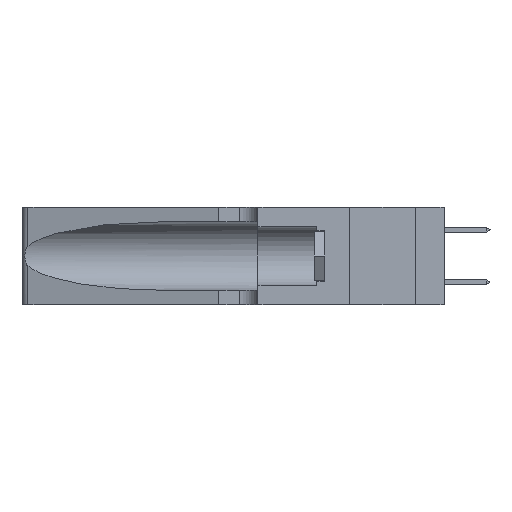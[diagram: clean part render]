
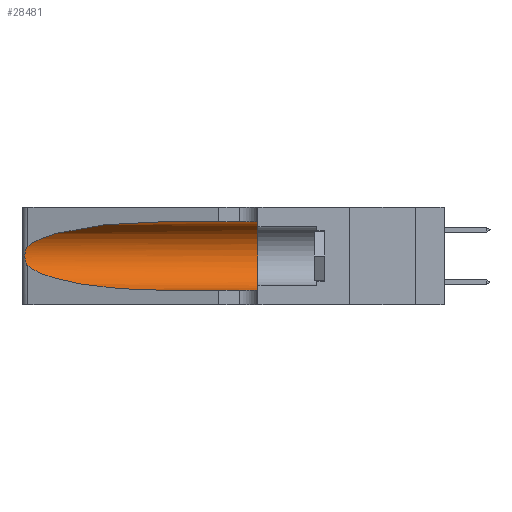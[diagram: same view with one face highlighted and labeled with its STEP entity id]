
A CAD part, left-side view. The second image highlights one B-rep face of the part: STEP entity #28481.
In plain terms, the highlighted cylindrical face has radius 3.308 mm (diameter 6.617 mm), a partial arc.
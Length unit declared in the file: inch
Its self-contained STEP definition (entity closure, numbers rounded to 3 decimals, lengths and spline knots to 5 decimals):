
#834 = DIRECTION ( 'NONE',  ( 0., -1., 0. ) ) ;
#1229 = VERTEX_POINT ( 'NONE', #6475 ) ;
#1246 = CARTESIAN_POINT ( 'NONE',  ( 0.25789, 1.23486, 0.15765 ) ) ;
#1828 = AXIS2_PLACEMENT_3D ( 'NONE', #7592, #24608, #10035 ) ;
#1978 = CARTESIAN_POINT ( 'NONE',  ( 0.1305, 0.35, 0.05475 ) ) ;
#2209 = DIRECTION ( 'NONE',  ( 0., 0., -1. ) ) ;
#2484 = AXIS2_PLACEMENT_3D ( 'NONE', #21669, #7104, #2209 ) ;
#3132 = CARTESIAN_POINT ( 'NONE',  ( 0.18966, 0.96281, 0.05475 ) ) ;
#3680 = CARTESIAN_POINT ( 'NONE',  ( 0.25555, 1.22993, 0.14849 ) ) ;
#4368 = VERTEX_POINT ( 'NONE', #24824 ) ;
#4526 = VECTOR ( 'NONE', #834, 39.37008 ) ;
#6027 = CARTESIAN_POINT ( 'NONE',  ( 0.25555, 1.22994, 0.2215 ) ) ;
#6126 = CARTESIAN_POINT ( 'NONE',  ( 0.25487, 1.22718, 0.22369 ) ) ;
#6475 = CARTESIAN_POINT ( 'NONE',  ( 0.25487, 1.22718, 0.22369 ) ) ;
#7104 = DIRECTION ( 'NONE',  ( 0., -1., 0. ) ) ;
#7253 = EDGE_CURVE ( 'NONE', #24562, #30715, #19856, .T. ) ;
#7592 = CARTESIAN_POINT ( 'NONE',  ( 0.1305, 0.35, 0.185 ) ) ;
#8226 = CARTESIAN_POINT ( 'NONE',  ( 0.25487, 1.22718, 0.14631 ) ) ;
#8473 = CARTESIAN_POINT ( 'NONE',  ( 0.25787, 1.23484, 0.2124 ) ) ;
#9405 = ORIENTED_EDGE ( 'NONE', *, *, #22318, .T. ) ;
#10035 = DIRECTION ( 'NONE',  ( 0., 0., 1. ) ) ;
#10339 = CARTESIAN_POINT ( 'NONE',  ( 0.1305, 0.72297, 0.31525 ) ) ;
#10905 = CARTESIAN_POINT ( 'NONE',  ( 0.26018, 1.23835, 0.19895 ) ) ;
#10991 = LINE ( 'NONE', #15040, #4526 ) ;
#11026 = CARTESIAN_POINT ( 'NONE',  ( 0.1305, 1.61858, 0.05475 ) ) ;
#12783 = CARTESIAN_POINT ( 'NONE',  ( 0.25487, 1.22718, 0.14631 ) ) ;
#12933 =( BOUNDED_CURVE ( )  B_SPLINE_CURVE ( 3, ( #12783, #24935, #3132, #20110 ),
 .UNSPECIFIED., .F., .F. ) 
 B_SPLINE_CURVE_WITH_KNOTS ( ( 4, 4 ),
 ( 3.44316, 4.71239 ),
 .UNSPECIFIED. ) 
 CURVE ( )  GEOMETRIC_REPRESENTATION_ITEM ( )  RATIONAL_B_SPLINE_CURVE ( ( 1., 0.87, 0.87, 1. ) ) 
 REPRESENTATION_ITEM ( '' )  );
#13247 = ORIENTED_EDGE ( 'NONE', *, *, #28868, .T. ) ;
#13335 = CARTESIAN_POINT ( 'NONE',  ( 0.26075, 1.23896, 0.178 ) ) ;
#13564 = EDGE_CURVE ( 'NONE', #16628, #24562, #10991, .T. ) ;
#15019 = LINE ( 'NONE', #11026, #21523 ) ;
#15040 = CARTESIAN_POINT ( 'NONE',  ( 0.1305, 1.61858, 0.31525 ) ) ;
#15261 = ORIENTED_EDGE ( 'NONE', *, *, #13564, .F. ) ;
#15773 = CARTESIAN_POINT ( 'NONE',  ( 0.18966, 0.96281, 0.31525 ) ) ;
#15777 = CARTESIAN_POINT ( 'NONE',  ( 0.25856, 1.23593, 0.16098 ) ) ;
#15968 = ORIENTED_EDGE ( 'NONE', *, *, #7253, .F. ) ;
#16098 = EDGE_CURVE ( 'NONE', #16628, #1229, #24274, .T. ) ;
#16628 = VERTEX_POINT ( 'NONE', #10339 ) ;
#18200 = CARTESIAN_POINT ( 'NONE',  ( 0.1305, 0.72297, 0.31525 ) ) ;
#18204 = CARTESIAN_POINT ( 'NONE',  ( 0.25639, 1.23186, 0.15144 ) ) ;
#18394 = CARTESIAN_POINT ( 'NONE',  ( 0.1305, 0.35, 0.31525 ) ) ;
#19856 = CIRCLE ( 'NONE', #1828, 0.13025 ) ;
#20110 = CARTESIAN_POINT ( 'NONE',  ( 0.1305, 0.72297, 0.05475 ) ) ;
#20555 = CARTESIAN_POINT ( 'NONE',  ( 0.25487, 1.22718, 0.22369 ) ) ;
#20663 = CARTESIAN_POINT ( 'NONE',  ( 0.2373, 1.15595, 0.28018 ) ) ;
#20665 = CARTESIAN_POINT ( 'NONE',  ( 0.25487, 1.22718, 0.14631 ) ) ;
#20749 = EDGE_CURVE ( 'NONE', #31088, #4368, #12933, .T. ) ;
#21165 = ORIENTED_EDGE ( 'NONE', *, *, #20749, .T. ) ;
#21425 = FACE_OUTER_BOUND ( 'NONE', #31111, .T. ) ;
#21523 = VECTOR ( 'NONE', #30501, 39.37008 ) ;
#21669 = CARTESIAN_POINT ( 'NONE',  ( 0.1305, 1.61858, 0.185 ) ) ;
#22318 = EDGE_CURVE ( 'NONE', #4368, #30715, #15019, .T. ) ;
#23030 = CARTESIAN_POINT ( 'NONE',  ( 0.25639, 1.23184, 0.21858 ) ) ;
#24274 =( BOUNDED_CURVE ( )  B_SPLINE_CURVE ( 3, ( #18200, #15773, #20663, #6126 ),
 .UNSPECIFIED., .F., .F. ) 
 B_SPLINE_CURVE_WITH_KNOTS ( ( 4, 4 ),
 ( 1.5708, 2.84003 ),
 .UNSPECIFIED. ) 
 CURVE ( )  GEOMETRIC_REPRESENTATION_ITEM ( )  RATIONAL_B_SPLINE_CURVE ( ( 1., 0.87, 0.87, 1. ) ) 
 REPRESENTATION_ITEM ( '' )  );
#24562 = VERTEX_POINT ( 'NONE', #18394 ) ;
#24608 = DIRECTION ( 'NONE',  ( 0., 1., 0. ) ) ;
#24824 = CARTESIAN_POINT ( 'NONE',  ( 0.1305, 0.72297, 0.05475 ) ) ;
#24935 = CARTESIAN_POINT ( 'NONE',  ( 0.2373, 1.15595, 0.08982 ) ) ;
#25500 = CARTESIAN_POINT ( 'NONE',  ( 0.25854, 1.2359, 0.20912 ) ) ;
#27130 = CYLINDRICAL_SURFACE ( 'NONE', #2484, 0.13025 ) ;
#27585 = B_SPLINE_CURVE_WITH_KNOTS ( 'NONE', 3,
 ( #20555, #6027, #23030, #8473, #25500, #10905, #27919, #13335, #30380, #15777, #1246, #18204, #3680, #20665 ),
 .UNSPECIFIED., .F., .F.,
 ( 4, 2, 2, 2, 2, 2, 4 ),
 ( 0., 0.00027, 0.00053, 0.00107, 0.0016, 0.00187, 0.00214 ),
 .UNSPECIFIED. ) ;
#27919 = CARTESIAN_POINT ( 'NONE',  ( 0.26075, 1.23896, 0.19203 ) ) ;
#28396 = ORIENTED_EDGE ( 'NONE', *, *, #16098, .T. ) ;
#28481 = ADVANCED_FACE ( 'NONE', ( #21425 ), #27130, .F. ) ;
#28868 = EDGE_CURVE ( 'NONE', #1229, #31088, #27585, .T. ) ;
#30380 = CARTESIAN_POINT ( 'NONE',  ( 0.26017, 1.23833, 0.17102 ) ) ;
#30501 = DIRECTION ( 'NONE',  ( 0., -1., 0. ) ) ;
#30715 = VERTEX_POINT ( 'NONE', #1978 ) ;
#31088 = VERTEX_POINT ( 'NONE', #8226 ) ;
#31111 = EDGE_LOOP ( 'NONE', ( #28396, #13247, #21165, #9405, #15968, #15261 ) ) ;
